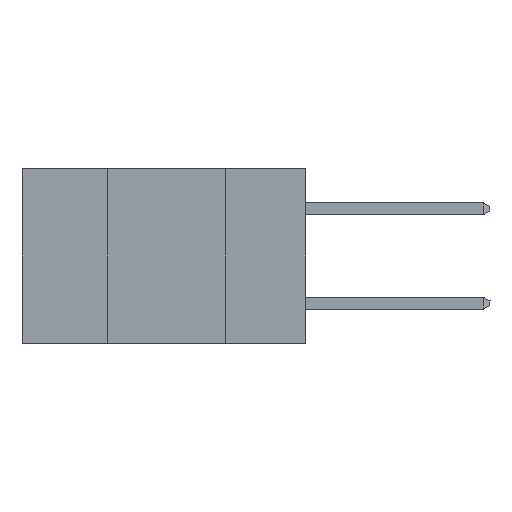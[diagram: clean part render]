
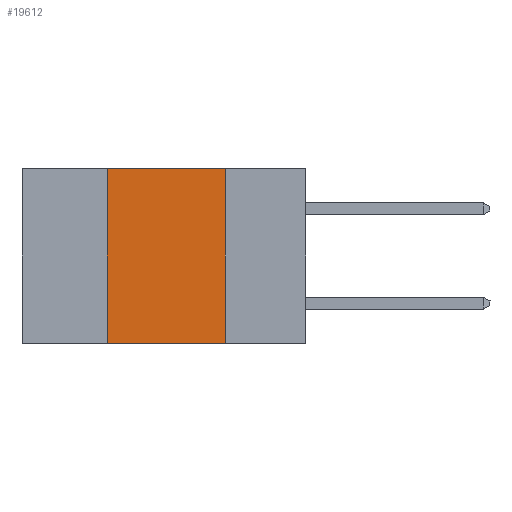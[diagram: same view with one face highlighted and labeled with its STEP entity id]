
A CAD part, left-side view. The second image highlights one B-rep face of the part: STEP entity #19612.
In plain terms, the highlighted planar face has unit normal (-1, 0, 0).
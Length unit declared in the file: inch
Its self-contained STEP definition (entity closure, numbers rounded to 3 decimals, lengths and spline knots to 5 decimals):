
#1178 = ORIENTED_EDGE ( 'NONE', *, *, #21396, .F. ) ;
#2212 = ORIENTED_EDGE ( 'NONE', *, *, #3042, .F. ) ;
#2453 = VERTEX_POINT ( 'NONE', #27503 ) ;
#3042 = EDGE_CURVE ( 'NONE', #18052, #4251, #25480, .T. ) ;
#3421 = CARTESIAN_POINT ( 'NONE',  ( 0., 0.17, -0.37 ) ) ;
#3553 = CARTESIAN_POINT ( 'NONE',  ( 0., 0.17, 0. ) ) ;
#4251 = VERTEX_POINT ( 'NONE', #23707 ) ;
#5386 = LINE ( 'NONE', #21140, #27214 ) ;
#5706 = EDGE_CURVE ( 'NONE', #4251, #21724, #7431, .T. ) ;
#6136 = CARTESIAN_POINT ( 'NONE',  ( 0., 0.6, -0.37 ) ) ;
#6323 = EDGE_CURVE ( 'NONE', #2453, #21724, #20919, .T. ) ;
#6988 = DIRECTION ( 'NONE',  ( 0., -1., 0. ) ) ;
#7431 = LINE ( 'NONE', #3553, #10017 ) ;
#10017 = VECTOR ( 'NONE', #26826, 39.37008 ) ;
#10922 = ORIENTED_EDGE ( 'NONE', *, *, #6323, .T. ) ;
#13424 = CARTESIAN_POINT ( 'NONE',  ( 0., 0.6, 0. ) ) ;
#13822 = VECTOR ( 'NONE', #6988, 39.37008 ) ;
#14615 = CARTESIAN_POINT ( 'NONE',  ( 0., 0.42, 0. ) ) ;
#14700 = VECTOR ( 'NONE', #22540, 39.37008 ) ;
#16353 = EDGE_LOOP ( 'NONE', ( #27242, #2212, #1178, #10922 ) ) ;
#16443 = CARTESIAN_POINT ( 'NONE',  ( 0., 0.6, 0. ) ) ;
#18052 = VERTEX_POINT ( 'NONE', #14615 ) ;
#19612 = ADVANCED_FACE ( 'NONE', ( #25453 ), #20540, .F. ) ;
#20540 = PLANE ( 'NONE',  #27298 ) ;
#20919 = LINE ( 'NONE', #6136, #14700 ) ;
#21140 = CARTESIAN_POINT ( 'NONE',  ( 0., 0.42, 0. ) ) ;
#21396 = EDGE_CURVE ( 'NONE', #2453, #18052, #5386, .T. ) ;
#21724 = VERTEX_POINT ( 'NONE', #3421 ) ;
#22540 = DIRECTION ( 'NONE',  ( 0., -1., 0. ) ) ;
#23707 = CARTESIAN_POINT ( 'NONE',  ( 0., 0.17, 0. ) ) ;
#24941 = DIRECTION ( 'NONE',  ( 0., 0., -1. ) ) ;
#25453 = FACE_OUTER_BOUND ( 'NONE', #16353, .T. ) ;
#25480 = LINE ( 'NONE', #16443, #13822 ) ;
#26826 = DIRECTION ( 'NONE',  ( 0., 0., -1. ) ) ;
#27214 = VECTOR ( 'NONE', #27824, 39.37008 ) ;
#27242 = ORIENTED_EDGE ( 'NONE', *, *, #5706, .F. ) ;
#27298 = AXIS2_PLACEMENT_3D ( 'NONE', #13424, #27551, #24941 ) ;
#27503 = CARTESIAN_POINT ( 'NONE',  ( 0., 0.42, -0.37 ) ) ;
#27551 = DIRECTION ( 'NONE',  ( 1., 0., 0. ) ) ;
#27824 = DIRECTION ( 'NONE',  ( 0., 0., 1. ) ) ;
